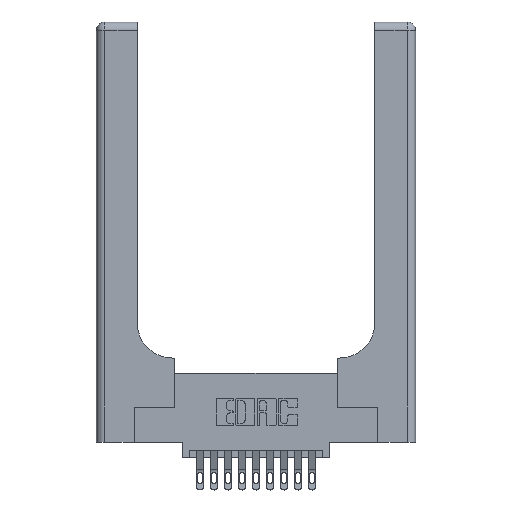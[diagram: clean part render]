
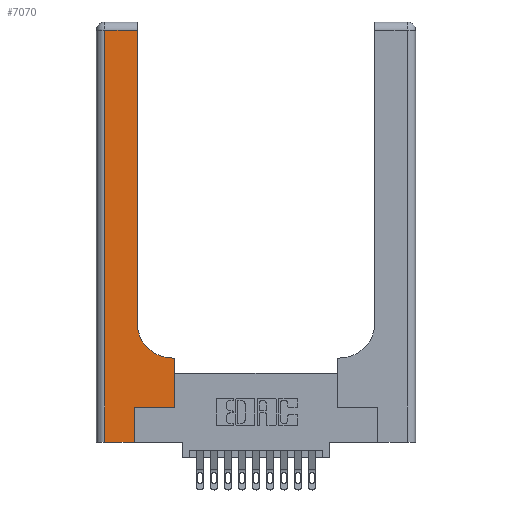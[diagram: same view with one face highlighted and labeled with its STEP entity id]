
A CAD part, top view. The second image highlights one B-rep face of the part: STEP entity #7070.
In plain terms, the highlighted planar face has unit normal (0, 0, 1).
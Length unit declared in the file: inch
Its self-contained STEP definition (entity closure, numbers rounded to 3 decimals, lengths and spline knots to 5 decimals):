
#218 = VECTOR ( 'NONE', #13175, 39.37008 ) ;
#730 = CARTESIAN_POINT ( 'NONE',  ( 0., 0., 0.37 ) ) ;
#945 = LINE ( 'NONE', #6276, #7740 ) ;
#1159 = CARTESIAN_POINT ( 'NONE',  ( 0.2915, 0.6, 0.37 ) ) ;
#1228 = DIRECTION ( 'NONE',  ( 0., 1., 0. ) ) ;
#2289 = LINE ( 'NONE', #6149, #9481 ) ;
#2342 = EDGE_CURVE ( 'NONE', #13305, #17135, #5585, .T. ) ;
#2605 = ORIENTED_EDGE ( 'NONE', *, *, #10362, .T. ) ;
#3107 = AXIS2_PLACEMENT_3D ( 'NONE', #14577, #8105, #17152 ) ;
#3280 = DIRECTION ( 'NONE',  ( -1., 0., 0. ) ) ;
#3477 = CARTESIAN_POINT ( 'NONE',  ( 0.2915, 0.85, 0.37 ) ) ;
#4344 = ORIENTED_EDGE ( 'NONE', *, *, #11176, .T. ) ;
#4599 = DIRECTION ( 'NONE',  ( 0., -1., 0. ) ) ;
#4681 = VERTEX_POINT ( 'NONE', #12341 ) ;
#4902 = CARTESIAN_POINT ( 'NONE',  ( 0.06, 2.94, 0.37 ) ) ;
#5585 = LINE ( 'NONE', #730, #6008 ) ;
#6008 = VECTOR ( 'NONE', #17069, 39.37008 ) ;
#6130 = EDGE_CURVE ( 'NONE', #8987, #13305, #16719, .T. ) ;
#6149 = CARTESIAN_POINT ( 'NONE',  ( 0.269, 0.25, 0.37 ) ) ;
#6276 = CARTESIAN_POINT ( 'NONE',  ( 0.269, 0., 0.37 ) ) ;
#6709 = CARTESIAN_POINT ( 'NONE',  ( 0.5585, 0.25, 0.37 ) ) ;
#6757 = PLANE ( 'NONE',  #3107 ) ;
#6783 = LINE ( 'NONE', #11948, #9894 ) ;
#7070 = ADVANCED_FACE ( 'NONE', ( #13682 ), #6757, .F. ) ;
#7086 = ORIENTED_EDGE ( 'NONE', *, *, #8986, .T. ) ;
#7087 = VECTOR ( 'NONE', #15815, 39.37008 ) ;
#7178 = DIRECTION ( 'NONE',  ( 0., 0., -1. ) ) ;
#7522 = ORIENTED_EDGE ( 'NONE', *, *, #13543, .T. ) ;
#7621 = DIRECTION ( 'NONE',  ( 0., 1., 0. ) ) ;
#7688 = EDGE_CURVE ( 'NONE', #4681, #14558, #9227, .T. ) ;
#7740 = VECTOR ( 'NONE', #7621, 39.37008 ) ;
#8105 = DIRECTION ( 'NONE',  ( 0., 0., -1. ) ) ;
#8216 = CARTESIAN_POINT ( 'NONE',  ( 0.269, 0.25, 0.37 ) ) ;
#8231 = VERTEX_POINT ( 'NONE', #8216 ) ;
#8676 = EDGE_LOOP ( 'NONE', ( #12824, #2605, #16638, #10204, #7086, #14036, #7522, #4344, #11819 ) ) ;
#8986 = EDGE_CURVE ( 'NONE', #17135, #8231, #945, .T. ) ;
#8987 = VERTEX_POINT ( 'NONE', #4902 ) ;
#9137 = VERTEX_POINT ( 'NONE', #13021 ) ;
#9227 = CIRCLE ( 'NONE', #9986, 0.25 ) ;
#9290 = VERTEX_POINT ( 'NONE', #14656 ) ;
#9481 = VECTOR ( 'NONE', #11391, 39.37008 ) ;
#9778 = LINE ( 'NONE', #6709, #7087 ) ;
#9779 = CARTESIAN_POINT ( 'NONE',  ( 0.269, 0., 0.37 ) ) ;
#9894 = VECTOR ( 'NONE', #1228, 39.37008 ) ;
#9986 = AXIS2_PLACEMENT_3D ( 'NONE', #14987, #7178, #16262 ) ;
#9988 = CARTESIAN_POINT ( 'NONE',  ( 0.5585, 0.25, 0.37 ) ) ;
#10204 = ORIENTED_EDGE ( 'NONE', *, *, #2342, .T. ) ;
#10213 = CARTESIAN_POINT ( 'NONE',  ( 0.06, 0., 0.37 ) ) ;
#10362 = EDGE_CURVE ( 'NONE', #9290, #8987, #13196, .T. ) ;
#10958 = LINE ( 'NONE', #1159, #218 ) ;
#11176 = EDGE_CURVE ( 'NONE', #9137, #4681, #10958, .T. ) ;
#11391 = DIRECTION ( 'NONE',  ( 1., 0., 0. ) ) ;
#11819 = ORIENTED_EDGE ( 'NONE', *, *, #7688, .T. ) ;
#11948 = CARTESIAN_POINT ( 'NONE',  ( 0.2915, 3., 0.37 ) ) ;
#12000 = VERTEX_POINT ( 'NONE', #9988 ) ;
#12341 = CARTESIAN_POINT ( 'NONE',  ( 0.5415, 0.6, 0.37 ) ) ;
#12491 = EDGE_CURVE ( 'NONE', #8231, #12000, #2289, .T. ) ;
#12589 = CARTESIAN_POINT ( 'NONE',  ( 0., 2.94, 0.37 ) ) ;
#12824 = ORIENTED_EDGE ( 'NONE', *, *, #16899, .T. ) ;
#13021 = CARTESIAN_POINT ( 'NONE',  ( 0.5585, 0.6, 0.37 ) ) ;
#13175 = DIRECTION ( 'NONE',  ( -1., 0., 0. ) ) ;
#13196 = LINE ( 'NONE', #12589, #16614 ) ;
#13305 = VERTEX_POINT ( 'NONE', #10213 ) ;
#13543 = EDGE_CURVE ( 'NONE', #12000, #9137, #9778, .T. ) ;
#13682 = FACE_OUTER_BOUND ( 'NONE', #8676, .T. ) ;
#13823 = CARTESIAN_POINT ( 'NONE',  ( 0.06, 3., 0.37 ) ) ;
#14036 = ORIENTED_EDGE ( 'NONE', *, *, #12491, .T. ) ;
#14558 = VERTEX_POINT ( 'NONE', #3477 ) ;
#14577 = CARTESIAN_POINT ( 'NONE',  ( 0., 3., 0.37 ) ) ;
#14656 = CARTESIAN_POINT ( 'NONE',  ( 0.2915, 2.94, 0.37 ) ) ;
#14987 = CARTESIAN_POINT ( 'NONE',  ( 0.5415, 0.85, 0.37 ) ) ;
#15815 = DIRECTION ( 'NONE',  ( 0., 1., 0. ) ) ;
#16262 = DIRECTION ( 'NONE',  ( 1., 0., 0. ) ) ;
#16614 = VECTOR ( 'NONE', #3280, 39.37008 ) ;
#16638 = ORIENTED_EDGE ( 'NONE', *, *, #6130, .T. ) ;
#16719 = LINE ( 'NONE', #13823, #17119 ) ;
#16899 = EDGE_CURVE ( 'NONE', #14558, #9290, #6783, .T. ) ;
#17069 = DIRECTION ( 'NONE',  ( 1., 0., 0. ) ) ;
#17119 = VECTOR ( 'NONE', #4599, 39.37008 ) ;
#17135 = VERTEX_POINT ( 'NONE', #9779 ) ;
#17152 = DIRECTION ( 'NONE',  ( -1., 0., 0. ) ) ;
